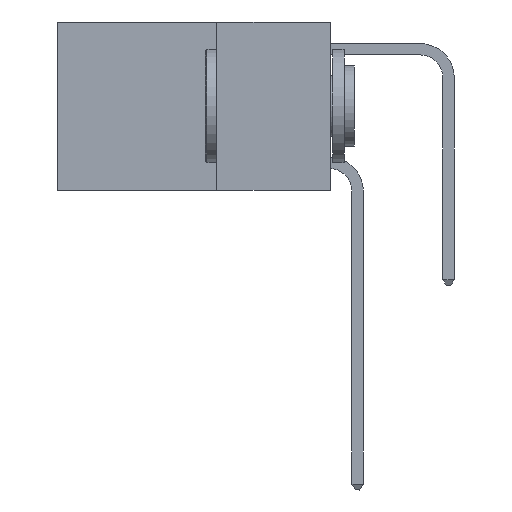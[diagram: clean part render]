
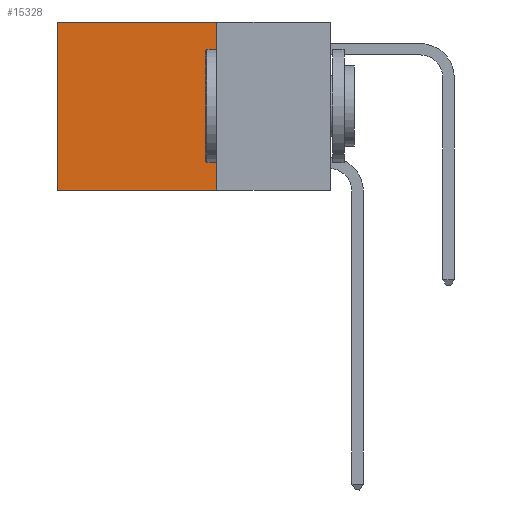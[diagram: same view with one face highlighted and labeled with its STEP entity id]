
A CAD part, left-side view. The second image highlights one B-rep face of the part: STEP entity #15328.
In plain terms, the highlighted planar face has unit normal (-1, 0, 0).
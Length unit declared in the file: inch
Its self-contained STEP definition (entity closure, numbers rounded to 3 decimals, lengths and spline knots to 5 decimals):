
#38 = CARTESIAN_POINT ( 'NONE',  ( 0.2625, 0.6, 0. ) ) ;
#940 = VERTEX_POINT ( 'NONE', #23757 ) ;
#1450 = LINE ( 'NONE', #17481, #11006 ) ;
#1466 = PLANE ( 'NONE',  #13577 ) ;
#1471 = EDGE_CURVE ( 'NONE', #32728, #27691, #28973, .T. ) ;
#2640 = VECTOR ( 'NONE', #10676, 39.37008 ) ;
#3095 = VERTEX_POINT ( 'NONE', #30049 ) ;
#5448 = LINE ( 'NONE', #38, #2640 ) ;
#8497 = EDGE_CURVE ( 'NONE', #3095, #940, #21112, .T. ) ;
#10676 = DIRECTION ( 'NONE',  ( 0., 0., -1. ) ) ;
#11006 = VECTOR ( 'NONE', #17658, 39.37008 ) ;
#13101 = DIRECTION ( 'NONE',  ( 0., 1., 0. ) ) ;
#13173 = EDGE_LOOP ( 'NONE', ( #20310, #28490, #23503, #23929 ) ) ;
#13322 = CARTESIAN_POINT ( 'NONE',  ( 0.2625, 0.6, 0. ) ) ;
#13577 = AXIS2_PLACEMENT_3D ( 'NONE', #27626, #14699, #30426 ) ;
#14699 = DIRECTION ( 'NONE',  ( 1., 0., 0. ) ) ;
#15328 = ADVANCED_FACE ( 'NONE', ( #20357 ), #1466, .F. ) ;
#15372 = CARTESIAN_POINT ( 'NONE',  ( 0.2625, 0.25, 0. ) ) ;
#17481 = CARTESIAN_POINT ( 'NONE',  ( 0.2625, 0.25, 0. ) ) ;
#17658 = DIRECTION ( 'NONE',  ( 0., 0., -1. ) ) ;
#18175 = DIRECTION ( 'NONE',  ( 0., 1., 0. ) ) ;
#18500 = CARTESIAN_POINT ( 'NONE',  ( 0.2625, 0.25, -0.37 ) ) ;
#20310 = ORIENTED_EDGE ( 'NONE', *, *, #20761, .T. ) ;
#20357 = FACE_OUTER_BOUND ( 'NONE', #13173, .T. ) ;
#20761 = EDGE_CURVE ( 'NONE', #27691, #940, #5448, .T. ) ;
#21036 = EDGE_CURVE ( 'NONE', #32728, #3095, #1450, .T. ) ;
#21112 = LINE ( 'NONE', #18500, #24874 ) ;
#23503 = ORIENTED_EDGE ( 'NONE', *, *, #21036, .F. ) ;
#23757 = CARTESIAN_POINT ( 'NONE',  ( 0.2625, 0.6, -0.37 ) ) ;
#23929 = ORIENTED_EDGE ( 'NONE', *, *, #1471, .T. ) ;
#24874 = VECTOR ( 'NONE', #13101, 39.37008 ) ;
#26155 = CARTESIAN_POINT ( 'NONE',  ( 0.2625, 0.25, 0. ) ) ;
#27626 = CARTESIAN_POINT ( 'NONE',  ( 0.2625, 0.25, 0. ) ) ;
#27691 = VERTEX_POINT ( 'NONE', #13322 ) ;
#28490 = ORIENTED_EDGE ( 'NONE', *, *, #8497, .F. ) ;
#28973 = LINE ( 'NONE', #15372, #30701 ) ;
#30049 = CARTESIAN_POINT ( 'NONE',  ( 0.2625, 0.25, -0.37 ) ) ;
#30426 = DIRECTION ( 'NONE',  ( 0., 0., -1. ) ) ;
#30701 = VECTOR ( 'NONE', #18175, 39.37008 ) ;
#32728 = VERTEX_POINT ( 'NONE', #26155 ) ;
